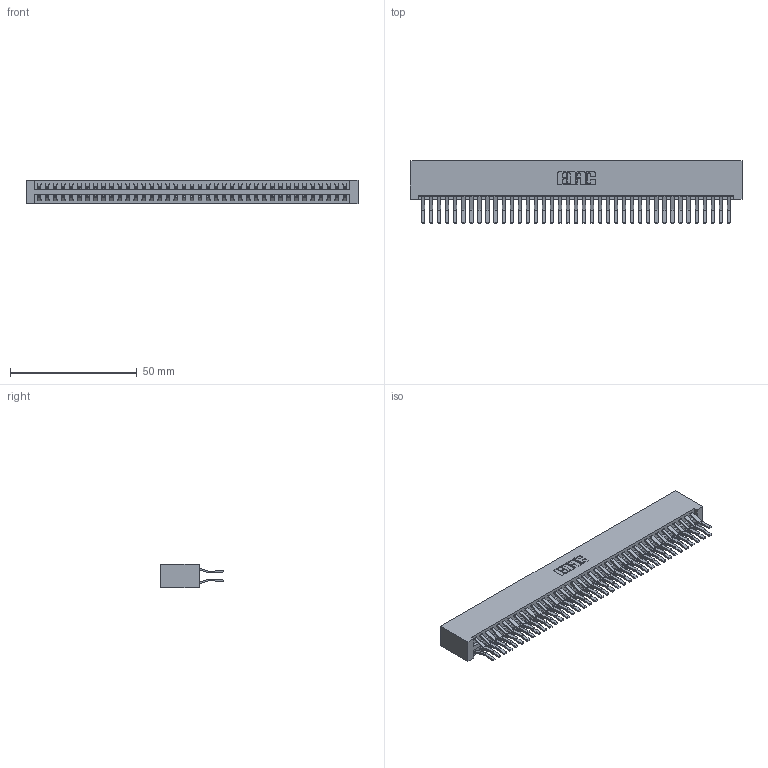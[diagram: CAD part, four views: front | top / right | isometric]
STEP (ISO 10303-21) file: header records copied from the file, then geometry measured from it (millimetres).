
FILE_DESCRIPTION (( 'STEP AP203' ), '1' );
FILE_NAME ('346-078-560-201.STEP', '2022-05-25T14:54:52', ( '' ), ( '' ), 'SwSTEP 2.0', 'SolidWorks 2020', '' );
FILE_SCHEMA (( 'CONFIG_CONTROL_DESIGN' ));
Length unit declared in the file: inch
Products named in the file (3): 345-292-001_560 Tail; 346-078-560-201; 346 Part_No Mounting Lugs
Assembly tree (79 placements, depth 2):
  346-078-560-201
    346 Part_No Mounting Lugs
    345-292-001_560 Tail  x78
Bounding box: 131.06 x 24.78 x 9.4 mm (x, y, z)
Volume: 13841.6 mm3; surface area: 20506.3 mm2
Topology: 79 solids, 79 shells, 4326 faces, 12863 edges, 8470 vertices
Faces by surface type: plane 2802, cylinder 1524
Entity records: 25667 total; most frequent: CARTESIAN_POINT 4232, ORIENTED_EDGE 4166, DIRECTION 3779, EDGE_CURVE 2083, VECTOR 1799, LINE 1799, VERTEX_POINT 1386, AXIS2_PLACEMENT_3D 990
